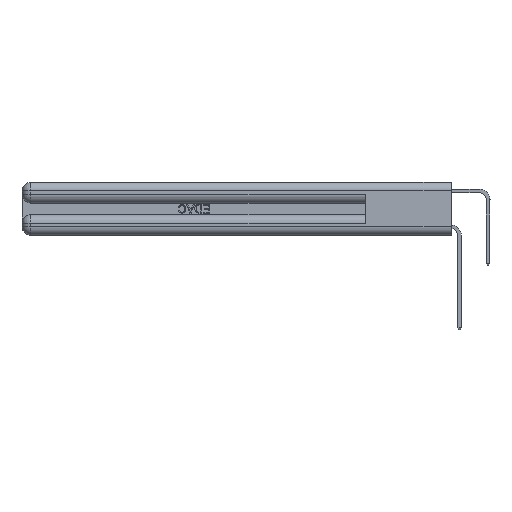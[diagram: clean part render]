
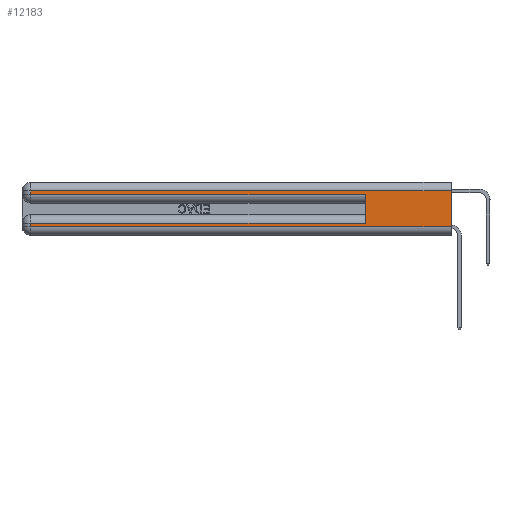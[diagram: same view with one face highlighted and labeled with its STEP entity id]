
A CAD part, left-side view. The second image highlights one B-rep face of the part: STEP entity #12183.
In plain terms, the highlighted planar face has unit normal (-1, 0, 0).
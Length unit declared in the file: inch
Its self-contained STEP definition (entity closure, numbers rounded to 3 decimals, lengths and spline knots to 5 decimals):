
#688 = CARTESIAN_POINT ( 'NONE',  ( 0., 2.94, 0.285 ) ) ;
#2171 = DIRECTION ( 'NONE',  ( 0., 0., -1. ) ) ;
#2554 = ORIENTED_EDGE ( 'NONE', *, *, #19529, .T. ) ;
#2629 = PLANE ( 'NONE',  #13573 ) ;
#3508 = LINE ( 'NONE', #14258, #11239 ) ;
#3946 = LINE ( 'NONE', #11235, #12616 ) ;
#4076 = LINE ( 'NONE', #14880, #29847 ) ;
#5140 = ORIENTED_EDGE ( 'NONE', *, *, #7060, .F. ) ;
#5195 = LINE ( 'NONE', #28992, #27527 ) ;
#6496 = LINE ( 'NONE', #30982, #13002 ) ;
#6570 = DIRECTION ( 'NONE',  ( 0., -1., 0. ) ) ;
#7060 = EDGE_CURVE ( 'NONE', #31416, #23161, #18707, .T. ) ;
#7406 = VECTOR ( 'NONE', #20536, 39.37008 ) ;
#7572 = ORIENTED_EDGE ( 'NONE', *, *, #33545, .T. ) ;
#8516 = CARTESIAN_POINT ( 'NONE',  ( 0., 2.94, 0.085 ) ) ;
#9642 = EDGE_CURVE ( 'NONE', #31416, #26069, #4076, .T. ) ;
#10389 = VERTEX_POINT ( 'NONE', #688 ) ;
#11235 = CARTESIAN_POINT ( 'NONE',  ( 0., 0.6, 0.145 ) ) ;
#11239 = VECTOR ( 'NONE', #24902, 39.37008 ) ;
#11561 = ORIENTED_EDGE ( 'NONE', *, *, #26248, .T. ) ;
#12183 = ADVANCED_FACE ( 'NONE', ( #14697 ), #2629, .F. ) ;
#12616 = VECTOR ( 'NONE', #32819, 39.37008 ) ;
#13002 = VECTOR ( 'NONE', #33968, 39.37008 ) ;
#13545 = DIRECTION ( 'NONE',  ( 1., 0., 0. ) ) ;
#13573 = AXIS2_PLACEMENT_3D ( 'NONE', #26716, #13545, #2171 ) ;
#14258 = CARTESIAN_POINT ( 'NONE',  ( 0., 2.94, 0.37 ) ) ;
#14697 = FACE_OUTER_BOUND ( 'NONE', #30175, .T. ) ;
#14880 = CARTESIAN_POINT ( 'NONE',  ( 0., 0., 0.31 ) ) ;
#15184 = EDGE_CURVE ( 'NONE', #28310, #29336, #3946, .T. ) ;
#16194 = ORIENTED_EDGE ( 'NONE', *, *, #26508, .T. ) ;
#16517 = CARTESIAN_POINT ( 'NONE',  ( 0., 0.6, 0.285 ) ) ;
#17123 = CARTESIAN_POINT ( 'NONE',  ( 0., 0., 0.31 ) ) ;
#17527 = CARTESIAN_POINT ( 'NONE',  ( 0., 0., 0.06 ) ) ;
#17942 = VERTEX_POINT ( 'NONE', #24205 ) ;
#18514 = CARTESIAN_POINT ( 'NONE',  ( 0., 0.6, 0.085 ) ) ;
#18707 = LINE ( 'NONE', #24238, #26384 ) ;
#18709 = LINE ( 'NONE', #17527, #27232 ) ;
#19529 = EDGE_CURVE ( 'NONE', #17942, #23161, #18709, .T. ) ;
#20065 = CARTESIAN_POINT ( 'NONE',  ( 0., 2.94, 0.31 ) ) ;
#20187 = CARTESIAN_POINT ( 'NONE',  ( 0., 0., 0.085 ) ) ;
#20536 = DIRECTION ( 'NONE',  ( 0., 1., 0. ) ) ;
#22188 = ORIENTED_EDGE ( 'NONE', *, *, #15184, .F. ) ;
#22206 = VERTEX_POINT ( 'NONE', #8516 ) ;
#23161 = VERTEX_POINT ( 'NONE', #34411 ) ;
#24205 = CARTESIAN_POINT ( 'NONE',  ( 0., 2.94, 0.06 ) ) ;
#24238 = CARTESIAN_POINT ( 'NONE',  ( 0., 0., 0.37 ) ) ;
#24450 = DIRECTION ( 'NONE',  ( 0., 0., -1. ) ) ;
#24902 = DIRECTION ( 'NONE',  ( 0., 0., -1. ) ) ;
#26069 = VERTEX_POINT ( 'NONE', #20065 ) ;
#26248 = EDGE_CURVE ( 'NONE', #28310, #22206, #27964, .T. ) ;
#26384 = VECTOR ( 'NONE', #26869, 39.37008 ) ;
#26508 = EDGE_CURVE ( 'NONE', #26069, #10389, #5195, .T. ) ;
#26569 = EDGE_CURVE ( 'NONE', #22206, #17942, #3508, .T. ) ;
#26716 = CARTESIAN_POINT ( 'NONE',  ( 0., 0., 0.37 ) ) ;
#26869 = DIRECTION ( 'NONE',  ( 0., 0., -1. ) ) ;
#26904 = ORIENTED_EDGE ( 'NONE', *, *, #9642, .T. ) ;
#27045 = DIRECTION ( 'NONE',  ( 0., 1., 0. ) ) ;
#27232 = VECTOR ( 'NONE', #6570, 39.37008 ) ;
#27527 = VECTOR ( 'NONE', #24450, 39.37008 ) ;
#27964 = LINE ( 'NONE', #20187, #7406 ) ;
#28310 = VERTEX_POINT ( 'NONE', #18514 ) ;
#28992 = CARTESIAN_POINT ( 'NONE',  ( 0., 2.94, 0.37 ) ) ;
#29336 = VERTEX_POINT ( 'NONE', #16517 ) ;
#29847 = VECTOR ( 'NONE', #27045, 39.37008 ) ;
#30175 = EDGE_LOOP ( 'NONE', ( #5140, #26904, #16194, #7572, #22188, #11561, #30252, #2554 ) ) ;
#30252 = ORIENTED_EDGE ( 'NONE', *, *, #26569, .T. ) ;
#30982 = CARTESIAN_POINT ( 'NONE',  ( 0., 0., 0.285 ) ) ;
#31416 = VERTEX_POINT ( 'NONE', #17123 ) ;
#32819 = DIRECTION ( 'NONE',  ( 0., 0., 1. ) ) ;
#33545 = EDGE_CURVE ( 'NONE', #10389, #29336, #6496, .T. ) ;
#33968 = DIRECTION ( 'NONE',  ( 0., -1., 0. ) ) ;
#34411 = CARTESIAN_POINT ( 'NONE',  ( 0., 0., 0.06 ) ) ;
